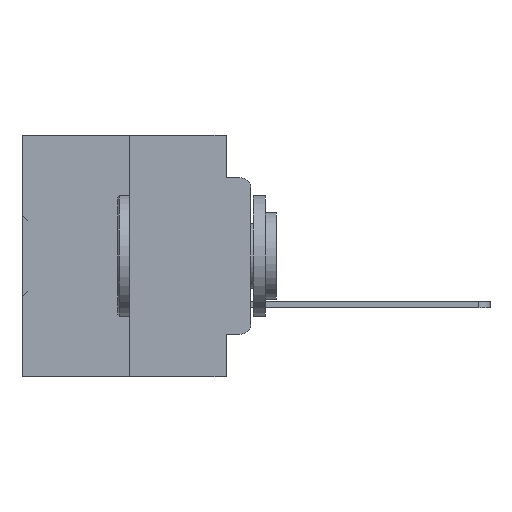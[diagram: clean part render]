
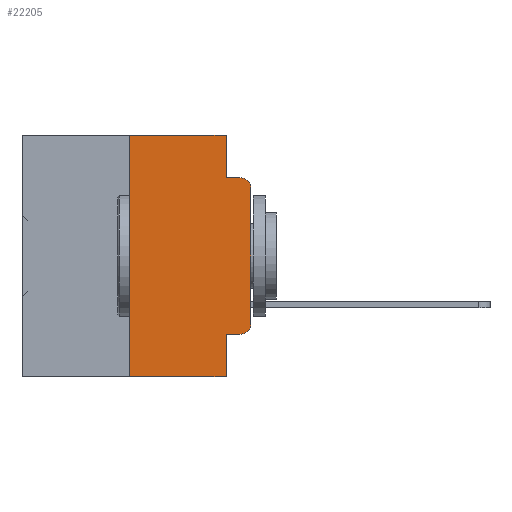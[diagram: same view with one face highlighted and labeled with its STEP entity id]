
A CAD part, left-side view. The second image highlights one B-rep face of the part: STEP entity #22205.
In plain terms, the highlighted planar face has unit normal (-1, 0, 0).
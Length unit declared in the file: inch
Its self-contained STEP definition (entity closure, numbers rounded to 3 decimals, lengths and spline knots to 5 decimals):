
#302 = CARTESIAN_POINT ( 'NONE',  ( 0., 0.25, 0. ) ) ;
#854 = VERTEX_POINT ( 'NONE', #302 ) ;
#1053 = CARTESIAN_POINT ( 'NONE',  ( 0., 0.02, -0.1085 ) ) ;
#1095 = ORIENTED_EDGE ( 'NONE', *, *, #29149, .T. ) ;
#2446 = VERTEX_POINT ( 'NONE', #3367 ) ;
#3367 = CARTESIAN_POINT ( 'NONE',  ( 0., 0.051, -0.4115 ) ) ;
#3628 = ORIENTED_EDGE ( 'NONE', *, *, #8224, .F. ) ;
#3814 = CARTESIAN_POINT ( 'NONE',  ( 0., 0.473, 0. ) ) ;
#4307 = DIRECTION ( 'NONE',  ( 0., 0., -1. ) ) ;
#4558 = VECTOR ( 'NONE', #26946, 39.37008 ) ;
#5464 = CARTESIAN_POINT ( 'NONE',  ( 0., 0.02, -0.0885 ) ) ;
#5971 = VECTOR ( 'NONE', #37238, 39.37008 ) ;
#6413 = AXIS2_PLACEMENT_3D ( 'NONE', #1053, #22808, #4307 ) ;
#7651 = ORIENTED_EDGE ( 'NONE', *, *, #34939, .F. ) ;
#8224 = EDGE_CURVE ( 'NONE', #26344, #31691, #9421, .T. ) ;
#8961 = CARTESIAN_POINT ( 'NONE',  ( 0., 0.25, 0. ) ) ;
#9130 = ORIENTED_EDGE ( 'NONE', *, *, #13102, .F. ) ;
#9421 = LINE ( 'NONE', #32657, #31376 ) ;
#9688 = VERTEX_POINT ( 'NONE', #18906 ) ;
#9938 = CARTESIAN_POINT ( 'NONE',  ( 0., 0.051, -0.0885 ) ) ;
#10282 = DIRECTION ( 'NONE',  ( 1., 0., 0. ) ) ;
#11109 = VECTOR ( 'NONE', #27695, 39.37008 ) ;
#11148 = DIRECTION ( 'NONE',  ( -1., 0., 0. ) ) ;
#12052 = DIRECTION ( 'NONE',  ( 0., 0., 1. ) ) ;
#12256 = CIRCLE ( 'NONE', #29909, 0.02 ) ;
#12893 = VERTEX_POINT ( 'NONE', #5464 ) ;
#13102 = EDGE_CURVE ( 'NONE', #31691, #12893, #26540, .T. ) ;
#13173 = LINE ( 'NONE', #8961, #23023 ) ;
#13214 = CARTESIAN_POINT ( 'NONE',  ( 0., 0., -0.1085 ) ) ;
#14069 = ORIENTED_EDGE ( 'NONE', *, *, #22577, .F. ) ;
#14645 = CARTESIAN_POINT ( 'NONE',  ( 0., 0.25, -0.5 ) ) ;
#15040 = ORIENTED_EDGE ( 'NONE', *, *, #16111, .T. ) ;
#15174 = CARTESIAN_POINT ( 'NONE',  ( 0., 0.473, 0. ) ) ;
#15396 = EDGE_LOOP ( 'NONE', ( #15480, #31127, #9130, #3628, #20210, #14069, #15040, #7651, #31586, #1095 ) ) ;
#15480 = ORIENTED_EDGE ( 'NONE', *, *, #31628, .T. ) ;
#15621 = VECTOR ( 'NONE', #33716, 39.37008 ) ;
#16111 = EDGE_CURVE ( 'NONE', #37095, #23450, #38912, .T. ) ;
#16587 = DIRECTION ( 'NONE',  ( 0., 0., -1. ) ) ;
#17451 = LINE ( 'NONE', #19517, #25350 ) ;
#18420 = FACE_OUTER_BOUND ( 'NONE', #15396, .T. ) ;
#18730 = VECTOR ( 'NONE', #30820, 39.37008 ) ;
#18906 = CARTESIAN_POINT ( 'NONE',  ( 0., 0.02, -0.4115 ) ) ;
#19235 = LINE ( 'NONE', #21833, #11109 ) ;
#19267 = CARTESIAN_POINT ( 'NONE',  ( 0., 0.051, -0.0885 ) ) ;
#19392 = PLANE ( 'NONE',  #28528 ) ;
#19517 = CARTESIAN_POINT ( 'NONE',  ( 0., 0.051, 0. ) ) ;
#20210 = ORIENTED_EDGE ( 'NONE', *, *, #36515, .F. ) ;
#20447 = EDGE_CURVE ( 'NONE', #2446, #9688, #22357, .T. ) ;
#21833 = CARTESIAN_POINT ( 'NONE',  ( 0., 0., 0. ) ) ;
#22205 = ADVANCED_FACE ( 'NONE', ( #18420 ), #19392, .F. ) ;
#22357 = LINE ( 'NONE', #34309, #5971 ) ;
#22577 = EDGE_CURVE ( 'NONE', #37095, #854, #13173, .T. ) ;
#22808 = DIRECTION ( 'NONE',  ( -1., 0., 0. ) ) ;
#23023 = VECTOR ( 'NONE', #12052, 39.37008 ) ;
#23450 = VERTEX_POINT ( 'NONE', #30261 ) ;
#24066 = DIRECTION ( 'NONE',  ( 0., 0., -1. ) ) ;
#25350 = VECTOR ( 'NONE', #16587, 39.37008 ) ;
#26344 = VERTEX_POINT ( 'NONE', #36762 ) ;
#26540 = LINE ( 'NONE', #9938, #18730 ) ;
#26946 = DIRECTION ( 'NONE',  ( 0., -1., 0. ) ) ;
#27695 = DIRECTION ( 'NONE',  ( 0., 0., 1. ) ) ;
#28421 = CIRCLE ( 'NONE', #6413, 0.02 ) ;
#28528 = AXIS2_PLACEMENT_3D ( 'NONE', #3814, #10282, #31117 ) ;
#28975 = CARTESIAN_POINT ( 'NONE',  ( 0., 0.02, -0.3915 ) ) ;
#29149 = EDGE_CURVE ( 'NONE', #9688, #35496, #12256, .T. ) ;
#29909 = AXIS2_PLACEMENT_3D ( 'NONE', #28975, #11148, #31882 ) ;
#30261 = CARTESIAN_POINT ( 'NONE',  ( 0., 0.051, -0.5 ) ) ;
#30820 = DIRECTION ( 'NONE',  ( 0., -1., 0. ) ) ;
#30845 = CARTESIAN_POINT ( 'NONE',  ( 0., 0.473, -0.5 ) ) ;
#30936 = EDGE_CURVE ( 'NONE', #34249, #12893, #28421, .T. ) ;
#31117 = DIRECTION ( 'NONE',  ( 0., 0., -1. ) ) ;
#31127 = ORIENTED_EDGE ( 'NONE', *, *, #30936, .T. ) ;
#31376 = VECTOR ( 'NONE', #24066, 39.37008 ) ;
#31586 = ORIENTED_EDGE ( 'NONE', *, *, #20447, .T. ) ;
#31628 = EDGE_CURVE ( 'NONE', #35496, #34249, #19235, .T. ) ;
#31691 = VERTEX_POINT ( 'NONE', #19267 ) ;
#31882 = DIRECTION ( 'NONE',  ( 0., 0., -1. ) ) ;
#32657 = CARTESIAN_POINT ( 'NONE',  ( 0., 0.051, 0. ) ) ;
#33716 = DIRECTION ( 'NONE',  ( 0., -1., 0. ) ) ;
#33811 = CARTESIAN_POINT ( 'NONE',  ( 0., 0., -0.3915 ) ) ;
#34249 = VERTEX_POINT ( 'NONE', #13214 ) ;
#34309 = CARTESIAN_POINT ( 'NONE',  ( 0., 0.051, -0.4115 ) ) ;
#34939 = EDGE_CURVE ( 'NONE', #2446, #23450, #17451, .T. ) ;
#35496 = VERTEX_POINT ( 'NONE', #33811 ) ;
#36508 = LINE ( 'NONE', #15174, #4558 ) ;
#36515 = EDGE_CURVE ( 'NONE', #854, #26344, #36508, .T. ) ;
#36762 = CARTESIAN_POINT ( 'NONE',  ( 0., 0.051, 0. ) ) ;
#37095 = VERTEX_POINT ( 'NONE', #14645 ) ;
#37238 = DIRECTION ( 'NONE',  ( 0., -1., 0. ) ) ;
#38912 = LINE ( 'NONE', #30845, #15621 ) ;
